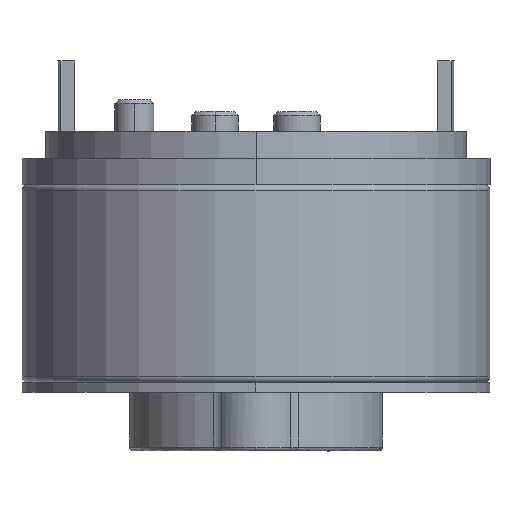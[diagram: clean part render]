
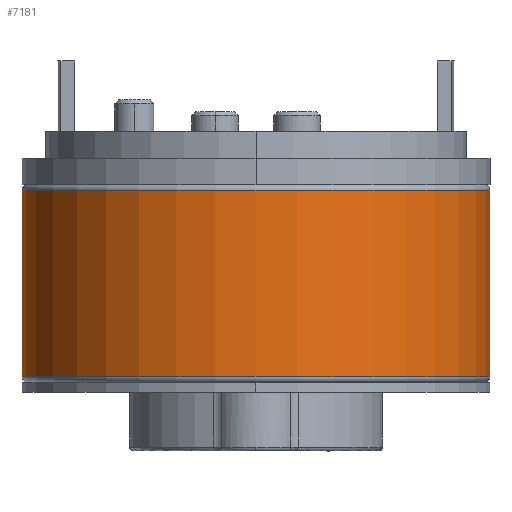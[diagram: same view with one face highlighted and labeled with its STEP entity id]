
A CAD part, left-side view. The second image highlights one B-rep face of the part: STEP entity #7181.
In plain terms, the highlighted cylindrical face has radius 6 mm (diameter 12 mm), a partial arc.
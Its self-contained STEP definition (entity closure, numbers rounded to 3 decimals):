
#256 = CARTESIAN_POINT ( 'NONE',  ( 0., -6., 6.4 ) ) ;
#762 = EDGE_CURVE ( 'NONE', #3832, #5962, #952, .T. ) ;
#924 = CARTESIAN_POINT ( 'NONE',  ( 0., 0., 3.069 ) ) ;
#952 = LINE ( 'NONE', #4622, #7304 ) ;
#1726 = ORIENTED_EDGE ( 'NONE', *, *, #3046, .F. ) ;
#2024 = CIRCLE ( 'NONE', #8401, 6. ) ;
#2291 = EDGE_LOOP ( 'NONE', ( #4814, #8691, #11494, #1726 ) ) ;
#2477 = VERTEX_POINT ( 'NONE', #256 ) ;
#3046 = EDGE_CURVE ( 'NONE', #10885, #2477, #3461, .T. ) ;
#3461 = LINE ( 'NONE', #7147, #3868 ) ;
#3462 = CARTESIAN_POINT ( 'NONE',  ( 0., 0., 11.18 ) ) ;
#3796 = CARTESIAN_POINT ( 'NONE',  ( 0., 0., 6.4 ) ) ;
#3832 = VERTEX_POINT ( 'NONE', #7292 ) ;
#3868 = VECTOR ( 'NONE', #11054, 1000. ) ;
#4592 = DIRECTION ( 'NONE',  ( 0., 0., -1. ) ) ;
#4622 = CARTESIAN_POINT ( 'NONE',  ( 0., 6., 3.069 ) ) ;
#4814 = ORIENTED_EDGE ( 'NONE', *, *, #5681, .T. ) ;
#5201 = CARTESIAN_POINT ( 'NONE',  ( 0., 6., 6.4 ) ) ;
#5517 = FACE_OUTER_BOUND ( 'NONE', #2291, .T. ) ;
#5681 = EDGE_CURVE ( 'NONE', #10885, #3832, #8632, .T. ) ;
#5962 = VERTEX_POINT ( 'NONE', #5201 ) ;
#6461 = EDGE_CURVE ( 'NONE', #2477, #5962, #2024, .T. ) ;
#7147 = CARTESIAN_POINT ( 'NONE',  ( 0., -6., 3.069 ) ) ;
#7150 = DIRECTION ( 'NONE',  ( 0., 0., -1. ) ) ;
#7181 = ADVANCED_FACE ( 'NONE', ( #5517 ), #9241, .T. ) ;
#7292 = CARTESIAN_POINT ( 'NONE',  ( 0., 6., 11.18 ) ) ;
#7304 = VECTOR ( 'NONE', #8340, 1000. ) ;
#7484 = DIRECTION ( 'NONE',  ( 0., 0., -1. ) ) ;
#8103 = CARTESIAN_POINT ( 'NONE',  ( 0., -6., 11.18 ) ) ;
#8313 = DIRECTION ( 'NONE',  ( 0., -1., 0. ) ) ;
#8340 = DIRECTION ( 'NONE',  ( 0., 0., -1. ) ) ;
#8401 = AXIS2_PLACEMENT_3D ( 'NONE', #3796, #7484, #11212 ) ;
#8476 = AXIS2_PLACEMENT_3D ( 'NONE', #3462, #7150, #10891 ) ;
#8632 = CIRCLE ( 'NONE', #8476, 6. ) ;
#8691 = ORIENTED_EDGE ( 'NONE', *, *, #762, .T. ) ;
#9241 = CYLINDRICAL_SURFACE ( 'NONE', #10304, 6. ) ;
#10304 = AXIS2_PLACEMENT_3D ( 'NONE', #924, #4592, #8313 ) ;
#10885 = VERTEX_POINT ( 'NONE', #8103 ) ;
#10891 = DIRECTION ( 'NONE',  ( 0.835, -0.55, 0. ) ) ;
#11054 = DIRECTION ( 'NONE',  ( 0., 0., -1. ) ) ;
#11212 = DIRECTION ( 'NONE',  ( 0.835, -0.55, 0. ) ) ;
#11494 = ORIENTED_EDGE ( 'NONE', *, *, #6461, .F. ) ;
